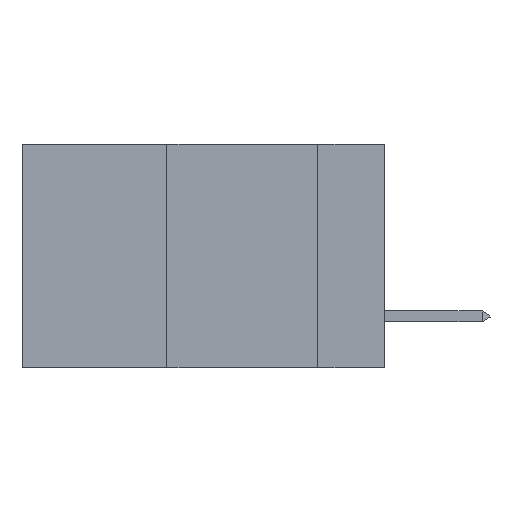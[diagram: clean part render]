
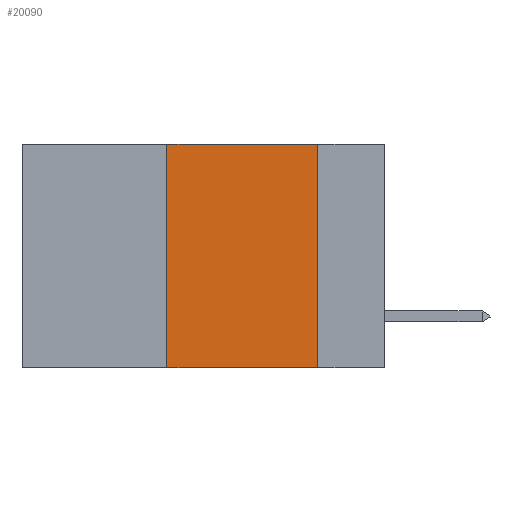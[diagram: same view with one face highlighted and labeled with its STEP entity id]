
A CAD part, left-side view. The second image highlights one B-rep face of the part: STEP entity #20090.
In plain terms, the highlighted planar face has unit normal (-1, 0, 0).
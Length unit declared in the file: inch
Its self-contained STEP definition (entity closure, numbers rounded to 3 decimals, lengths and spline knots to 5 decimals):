
#4 = DIRECTION ( 'NONE',  ( 0., 0., -1. ) ) ;
#634 = LINE ( 'NONE', #4796, #17900 ) ;
#1217 = VECTOR ( 'NONE', #25876, 39.37008 ) ;
#1697 = AXIS2_PLACEMENT_3D ( 'NONE', #13501, #7014, #4997 ) ;
#2528 = LINE ( 'NONE', #12914, #1217 ) ;
#2746 = CARTESIAN_POINT ( 'NONE',  ( 0., 0.6, -0.37 ) ) ;
#3650 = FACE_OUTER_BOUND ( 'NONE', #14388, .T. ) ;
#3812 = VECTOR ( 'NONE', #4, 39.37008 ) ;
#4017 = CARTESIAN_POINT ( 'NONE',  ( 0., 0.11, 0. ) ) ;
#4796 = CARTESIAN_POINT ( 'NONE',  ( 0., 0.36, 0. ) ) ;
#4874 = VERTEX_POINT ( 'NONE', #22033 ) ;
#4997 = DIRECTION ( 'NONE',  ( 0., 0., -1. ) ) ;
#5054 = DIRECTION ( 'NONE',  ( 0., -1., 0. ) ) ;
#5398 = VERTEX_POINT ( 'NONE', #23530 ) ;
#5870 = VERTEX_POINT ( 'NONE', #22056 ) ;
#6091 = LINE ( 'NONE', #12666, #3812 ) ;
#7014 = DIRECTION ( 'NONE',  ( 1., 0., 0. ) ) ;
#10061 = VERTEX_POINT ( 'NONE', #4017 ) ;
#12666 = CARTESIAN_POINT ( 'NONE',  ( 0., 0.11, 0. ) ) ;
#12914 = CARTESIAN_POINT ( 'NONE',  ( 0., 0.6, 0. ) ) ;
#13501 = CARTESIAN_POINT ( 'NONE',  ( 0., 0.6, 0. ) ) ;
#14097 = VECTOR ( 'NONE', #5054, 39.37008 ) ;
#14388 = EDGE_LOOP ( 'NONE', ( #19128, #22124, #14960, #22063 ) ) ;
#14960 = ORIENTED_EDGE ( 'NONE', *, *, #20552, .F. ) ;
#17485 = EDGE_CURVE ( 'NONE', #10061, #4874, #6091, .T. ) ;
#17900 = VECTOR ( 'NONE', #19646, 39.37008 ) ;
#19128 = ORIENTED_EDGE ( 'NONE', *, *, #17485, .F. ) ;
#19646 = DIRECTION ( 'NONE',  ( 0., 0., 1. ) ) ;
#20090 = ADVANCED_FACE ( 'NONE', ( #3650 ), #26280, .F. ) ;
#20552 = EDGE_CURVE ( 'NONE', #5398, #5870, #634, .T. ) ;
#22033 = CARTESIAN_POINT ( 'NONE',  ( 0., 0.11, -0.37 ) ) ;
#22056 = CARTESIAN_POINT ( 'NONE',  ( 0., 0.36, 0. ) ) ;
#22063 = ORIENTED_EDGE ( 'NONE', *, *, #22691, .T. ) ;
#22124 = ORIENTED_EDGE ( 'NONE', *, *, #22583, .F. ) ;
#22583 = EDGE_CURVE ( 'NONE', #5870, #10061, #2528, .T. ) ;
#22691 = EDGE_CURVE ( 'NONE', #5398, #4874, #25459, .T. ) ;
#23530 = CARTESIAN_POINT ( 'NONE',  ( 0., 0.36, -0.37 ) ) ;
#25459 = LINE ( 'NONE', #2746, #14097 ) ;
#25876 = DIRECTION ( 'NONE',  ( 0., -1., 0. ) ) ;
#26280 = PLANE ( 'NONE',  #1697 ) ;
